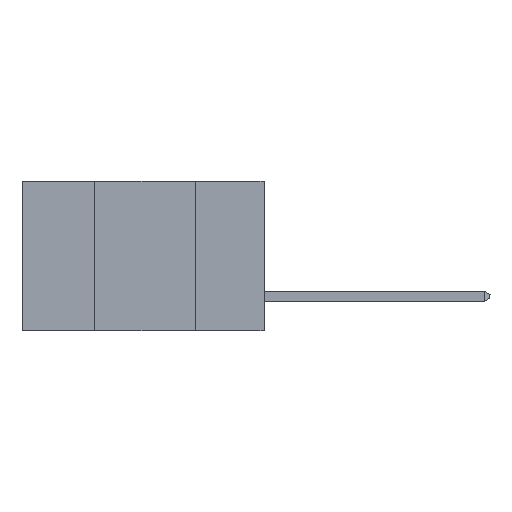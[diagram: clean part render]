
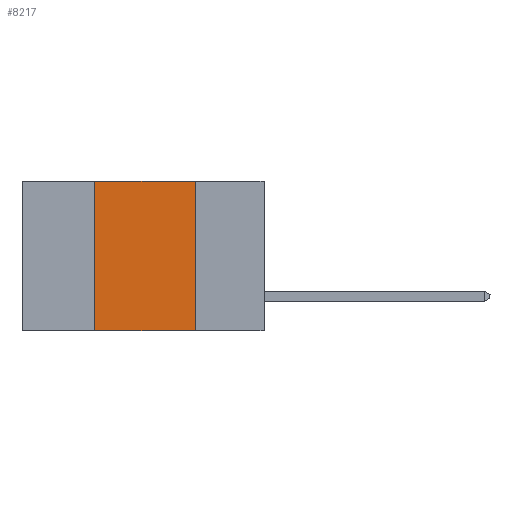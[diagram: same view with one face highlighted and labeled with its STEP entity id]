
A CAD part, left-side view. The second image highlights one B-rep face of the part: STEP entity #8217.
In plain terms, the highlighted planar face has unit normal (-1, 0, 0).
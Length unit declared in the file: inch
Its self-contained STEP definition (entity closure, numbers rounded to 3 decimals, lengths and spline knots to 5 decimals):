
#794 = VERTEX_POINT ( 'NONE', #6017 ) ;
#824 = CARTESIAN_POINT ( 'NONE',  ( 0., 0.42, 0. ) ) ;
#1319 = EDGE_CURVE ( 'NONE', #3949, #794, #2242, .T. ) ;
#1466 = ORIENTED_EDGE ( 'NONE', *, *, #8071, .F. ) ;
#1894 = DIRECTION ( 'NONE',  ( 1., 0., 0. ) ) ;
#1996 = ORIENTED_EDGE ( 'NONE', *, *, #10269, .F. ) ;
#2242 = LINE ( 'NONE', #2933, #7504 ) ;
#2399 = ORIENTED_EDGE ( 'NONE', *, *, #3643, .F. ) ;
#2769 = DIRECTION ( 'NONE',  ( 0., 0., -1. ) ) ;
#2933 = CARTESIAN_POINT ( 'NONE',  ( 0., 0.6, -0.37 ) ) ;
#2992 = LINE ( 'NONE', #824, #3875 ) ;
#3120 = CARTESIAN_POINT ( 'NONE',  ( 0., 0.6, 0. ) ) ;
#3362 = AXIS2_PLACEMENT_3D ( 'NONE', #5469, #1894, #2769 ) ;
#3643 = EDGE_CURVE ( 'NONE', #5402, #11573, #6609, .T. ) ;
#3834 = CARTESIAN_POINT ( 'NONE',  ( 0., 0.17, 0. ) ) ;
#3875 = VECTOR ( 'NONE', #7905, 39.37008 ) ;
#3949 = VERTEX_POINT ( 'NONE', #6529 ) ;
#4074 = DIRECTION ( 'NONE',  ( 0., -1., 0. ) ) ;
#4752 = ORIENTED_EDGE ( 'NONE', *, *, #1319, .T. ) ;
#5402 = VERTEX_POINT ( 'NONE', #5912 ) ;
#5462 = FACE_OUTER_BOUND ( 'NONE', #5899, .T. ) ;
#5469 = CARTESIAN_POINT ( 'NONE',  ( 0., 0.6, 0. ) ) ;
#5505 = CARTESIAN_POINT ( 'NONE',  ( 0., 0.17, 0. ) ) ;
#5899 = EDGE_LOOP ( 'NONE', ( #1466, #2399, #1996, #4752 ) ) ;
#5912 = CARTESIAN_POINT ( 'NONE',  ( 0., 0.42, 0. ) ) ;
#6017 = CARTESIAN_POINT ( 'NONE',  ( 0., 0.17, -0.37 ) ) ;
#6181 = VECTOR ( 'NONE', #8443, 39.37008 ) ;
#6391 = PLANE ( 'NONE',  #3362 ) ;
#6529 = CARTESIAN_POINT ( 'NONE',  ( 0., 0.42, -0.37 ) ) ;
#6609 = LINE ( 'NONE', #3120, #8322 ) ;
#7504 = VECTOR ( 'NONE', #10213, 39.37008 ) ;
#7905 = DIRECTION ( 'NONE',  ( 0., 0., 1. ) ) ;
#8071 = EDGE_CURVE ( 'NONE', #11573, #794, #11664, .T. ) ;
#8217 = ADVANCED_FACE ( 'NONE', ( #5462 ), #6391, .F. ) ;
#8322 = VECTOR ( 'NONE', #4074, 39.37008 ) ;
#8443 = DIRECTION ( 'NONE',  ( 0., 0., -1. ) ) ;
#10213 = DIRECTION ( 'NONE',  ( 0., -1., 0. ) ) ;
#10269 = EDGE_CURVE ( 'NONE', #3949, #5402, #2992, .T. ) ;
#11573 = VERTEX_POINT ( 'NONE', #5505 ) ;
#11664 = LINE ( 'NONE', #3834, #6181 ) ;
